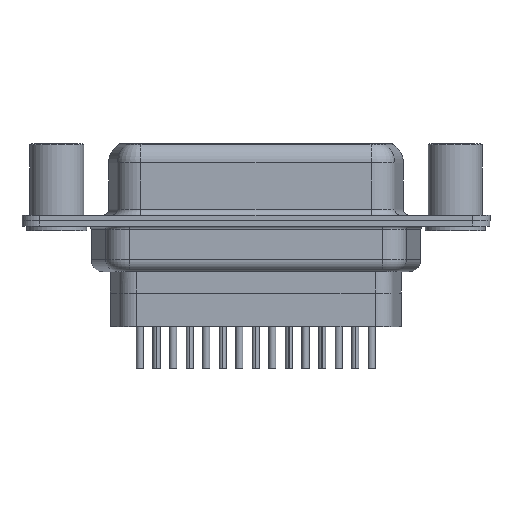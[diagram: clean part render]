
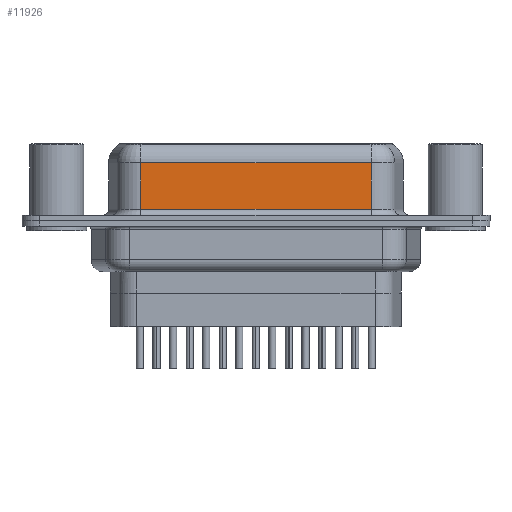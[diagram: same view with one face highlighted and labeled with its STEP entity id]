
A CAD part, front view. The second image highlights one B-rep face of the part: STEP entity #11926.
In plain terms, the highlighted planar face has unit normal (0, -1, 0).
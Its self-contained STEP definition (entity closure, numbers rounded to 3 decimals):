
#646 = EDGE_CURVE ( 'NONE', #4148, #16985, #20384, .T. ) ;
#1169 = ORIENTED_EDGE ( 'NONE', *, *, #19123, .T. ) ;
#2253 = CARTESIAN_POINT ( 'NONE',  ( 7.023, -3.95, 6.6 ) ) ;
#2651 = DIRECTION ( 'NONE',  ( 0., 0., -1. ) ) ;
#3168 = FACE_OUTER_BOUND ( 'NONE', #26091, .T. ) ;
#4148 = VERTEX_POINT ( 'NONE', #6968 ) ;
#5136 = EDGE_CURVE ( 'NONE', #24774, #4148, #21237, .T. ) ;
#5162 = PLANE ( 'NONE',  #14033 ) ;
#5382 = VECTOR ( 'NONE', #2651, 1000. ) ;
#5693 = VECTOR ( 'NONE', #24603, 1000. ) ;
#6000 = CARTESIAN_POINT ( 'NONE',  ( 26.297, -3.95, 0.95 ) ) ;
#6968 = CARTESIAN_POINT ( 'NONE',  ( 7.023, -3.95, 4.85 ) ) ;
#8618 = ORIENTED_EDGE ( 'NONE', *, *, #646, .T. ) ;
#10109 = CARTESIAN_POINT ( 'NONE',  ( 26.297, -3.95, 6.6 ) ) ;
#11227 = VECTOR ( 'NONE', #22870, 1000. ) ;
#11926 = ADVANCED_FACE ( 'NONE', ( #3168 ), #5162, .F. ) ;
#12276 = LINE ( 'NONE', #6000, #25224 ) ;
#13861 = VERTEX_POINT ( 'NONE', #14786 ) ;
#14033 = AXIS2_PLACEMENT_3D ( 'NONE', #23283, #15054, #25262 ) ;
#14786 = CARTESIAN_POINT ( 'NONE',  ( 26.297, -3.95, 0.95 ) ) ;
#15054 = DIRECTION ( 'NONE',  ( 0., 1., 0. ) ) ;
#16704 = ORIENTED_EDGE ( 'NONE', *, *, #19492, .F. ) ;
#16985 = VERTEX_POINT ( 'NONE', #17674 ) ;
#17674 = CARTESIAN_POINT ( 'NONE',  ( 7.023, -3.95, 0.95 ) ) ;
#18618 = ORIENTED_EDGE ( 'NONE', *, *, #5136, .T. ) ;
#19123 = EDGE_CURVE ( 'NONE', #16985, #13861, #12276, .T. ) ;
#19258 = CARTESIAN_POINT ( 'NONE',  ( 26.297, -3.95, 4.85 ) ) ;
#19492 = EDGE_CURVE ( 'NONE', #24774, #13861, #22617, .T. ) ;
#20384 = LINE ( 'NONE', #2253, #5382 ) ;
#21237 = LINE ( 'NONE', #19258, #11227 ) ;
#22617 = LINE ( 'NONE', #10109, #5693 ) ;
#22870 = DIRECTION ( 'NONE',  ( -1., 0., 0. ) ) ;
#23283 = CARTESIAN_POINT ( 'NONE',  ( 26.297, -3.95, 6.6 ) ) ;
#23589 = CARTESIAN_POINT ( 'NONE',  ( 26.297, -3.95, 4.85 ) ) ;
#24603 = DIRECTION ( 'NONE',  ( 0., 0., -1. ) ) ;
#24640 = DIRECTION ( 'NONE',  ( 1., 0., 0. ) ) ;
#24774 = VERTEX_POINT ( 'NONE', #23589 ) ;
#25224 = VECTOR ( 'NONE', #24640, 1000. ) ;
#25262 = DIRECTION ( 'NONE',  ( 0., 0., 1. ) ) ;
#26091 = EDGE_LOOP ( 'NONE', ( #16704, #18618, #8618, #1169 ) ) ;
